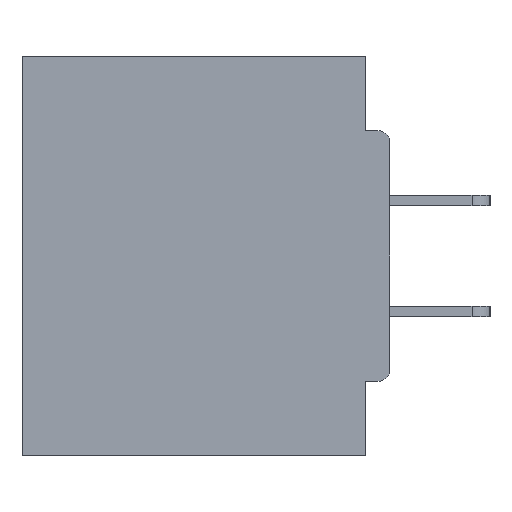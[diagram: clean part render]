
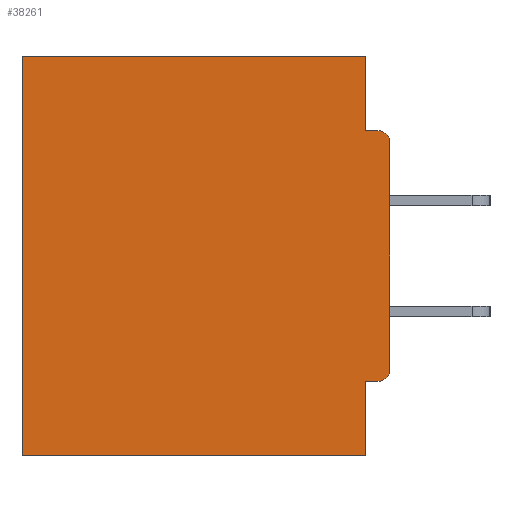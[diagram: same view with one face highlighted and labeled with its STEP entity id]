
A CAD part, left-side view. The second image highlights one B-rep face of the part: STEP entity #38261.
In plain terms, the highlighted planar face has unit normal (-1, 0, 0).
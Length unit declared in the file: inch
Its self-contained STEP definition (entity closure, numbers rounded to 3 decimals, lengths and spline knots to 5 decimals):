
#1 = CARTESIAN_POINT ( 'NONE',  ( 0.298, 0., 0. ) ) ;
#10 = ORIENTED_EDGE ( 'NONE', *, *, #27527, .F. ) ;
#19 = AXIS2_PLACEMENT_3D ( 'NONE', #25079, #4107, #12737 ) ;
#403 = VERTEX_POINT ( 'NONE', #8945 ) ;
#1099 = EDGE_CURVE ( 'NONE', #12573, #403, #3308, .T. ) ;
#2361 = CIRCLE ( 'NONE', #19, 0.015 ) ;
#2599 = VECTOR ( 'NONE', #16436, 39.37008 ) ;
#3308 = LINE ( 'NONE', #29332, #23283 ) ;
#3313 = DIRECTION ( 'NONE',  ( 1., 0., 0. ) ) ;
#4107 = DIRECTION ( 'NONE',  ( -1., 0., 0. ) ) ;
#4191 = LINE ( 'NONE', #11515, #24148 ) ;
#4206 = CARTESIAN_POINT ( 'NONE',  ( 0.298, 0.031, -0.4065 ) ) ;
#4776 = DIRECTION ( 'NONE',  ( 0., 0., -1. ) ) ;
#4802 = DIRECTION ( 'NONE',  ( -1., 0., 0. ) ) ;
#5469 = ORIENTED_EDGE ( 'NONE', *, *, #5647, .T. ) ;
#5568 = LINE ( 'NONE', #31179, #26936 ) ;
#5587 = VERTEX_POINT ( 'NONE', #21786 ) ;
#5647 = EDGE_CURVE ( 'NONE', #19175, #5587, #13406, .T. ) ;
#5949 = LINE ( 'NONE', #16168, #2599 ) ;
#6854 = ORIENTED_EDGE ( 'NONE', *, *, #15138, .T. ) ;
#6889 = DIRECTION ( 'NONE',  ( 0., 1., 0. ) ) ;
#8459 = DIRECTION ( 'NONE',  ( 0., 1., 0. ) ) ;
#8945 = CARTESIAN_POINT ( 'NONE',  ( 0.298, 0.031, -0.5 ) ) ;
#9092 = EDGE_CURVE ( 'NONE', #21730, #30964, #26271, .T. ) ;
#9103 = LINE ( 'NONE', #19027, #26215 ) ;
#9618 = CARTESIAN_POINT ( 'NONE',  ( 0.298, 0., 0. ) ) ;
#9807 = CARTESIAN_POINT ( 'NONE',  ( 0.298, 0.46, -0.5 ) ) ;
#10037 = CARTESIAN_POINT ( 'NONE',  ( 0.298, 0., -0.3915 ) ) ;
#10642 = VECTOR ( 'NONE', #24875, 39.37008 ) ;
#11515 = CARTESIAN_POINT ( 'NONE',  ( 0.298, 0., -0.5 ) ) ;
#11599 = EDGE_CURVE ( 'NONE', #403, #28120, #4191, .T. ) ;
#12137 = CARTESIAN_POINT ( 'NONE',  ( 0.298, 0.015, -0.0935 ) ) ;
#12368 = CARTESIAN_POINT ( 'NONE',  ( 0.298, 0.031, -0.0935 ) ) ;
#12519 = CARTESIAN_POINT ( 'NONE',  ( 0.298, 0.031, -0.5 ) ) ;
#12573 = VERTEX_POINT ( 'NONE', #4206 ) ;
#12737 = DIRECTION ( 'NONE',  ( 0., 0., -1. ) ) ;
#13051 = CARTESIAN_POINT ( 'NONE',  ( 0.298, 0.015, -0.4065 ) ) ;
#13172 = EDGE_CURVE ( 'NONE', #37526, #30964, #5568, .T. ) ;
#13406 = LINE ( 'NONE', #15814, #27646 ) ;
#13421 = ORIENTED_EDGE ( 'NONE', *, *, #32787, .F. ) ;
#14920 = LINE ( 'NONE', #12519, #10642 ) ;
#15113 = DIRECTION ( 'NONE',  ( 0., 0., -1. ) ) ;
#15138 = EDGE_CURVE ( 'NONE', #5587, #28120, #5949, .T. ) ;
#15471 = ORIENTED_EDGE ( 'NONE', *, *, #11599, .F. ) ;
#15814 = CARTESIAN_POINT ( 'NONE',  ( 0.298, 0., 0. ) ) ;
#16168 = CARTESIAN_POINT ( 'NONE',  ( 0.298, 0.46, 0. ) ) ;
#16307 = DIRECTION ( 'NONE',  ( 0., -1., 0. ) ) ;
#16319 = ORIENTED_EDGE ( 'NONE', *, *, #1099, .F. ) ;
#16436 = DIRECTION ( 'NONE',  ( 0., 0., -1. ) ) ;
#18049 = PLANE ( 'NONE',  #19138 ) ;
#18093 = ORIENTED_EDGE ( 'NONE', *, *, #9092, .T. ) ;
#18647 = FACE_OUTER_BOUND ( 'NONE', #21057, .T. ) ;
#19027 = CARTESIAN_POINT ( 'NONE',  ( 0.298, 0., -0.4065 ) ) ;
#19138 = AXIS2_PLACEMENT_3D ( 'NONE', #1, #3313, #15113 ) ;
#19175 = VERTEX_POINT ( 'NONE', #28108 ) ;
#19326 = VECTOR ( 'NONE', #24627, 39.37008 ) ;
#21057 = EDGE_LOOP ( 'NONE', ( #18093, #24665, #13421, #5469, #6854, #15471, #16319, #10, #34621, #32211 ) ) ;
#21522 = VERTEX_POINT ( 'NONE', #10037 ) ;
#21730 = VERTEX_POINT ( 'NONE', #32889 ) ;
#21786 = CARTESIAN_POINT ( 'NONE',  ( 0.298, 0.46, 0. ) ) ;
#23283 = VECTOR ( 'NONE', #4776, 39.37008 ) ;
#24148 = VECTOR ( 'NONE', #8459, 39.37008 ) ;
#24627 = DIRECTION ( 'NONE',  ( 0., 0., -1. ) ) ;
#24665 = ORIENTED_EDGE ( 'NONE', *, *, #13172, .F. ) ;
#24875 = DIRECTION ( 'NONE',  ( 0., 0., -1. ) ) ;
#25079 = CARTESIAN_POINT ( 'NONE',  ( 0.298, 0.015, -0.3915 ) ) ;
#26007 = LINE ( 'NONE', #9618, #19326 ) ;
#26215 = VECTOR ( 'NONE', #36690, 39.37008 ) ;
#26271 = CIRCLE ( 'NONE', #37431, 0.015 ) ;
#26512 = EDGE_CURVE ( 'NONE', #27689, #21522, #2361, .T. ) ;
#26936 = VECTOR ( 'NONE', #16307, 39.37008 ) ;
#27527 = EDGE_CURVE ( 'NONE', #27689, #12573, #9103, .T. ) ;
#27646 = VECTOR ( 'NONE', #6889, 39.37008 ) ;
#27689 = VERTEX_POINT ( 'NONE', #13051 ) ;
#28108 = CARTESIAN_POINT ( 'NONE',  ( 0.298, 0.031, 0. ) ) ;
#28120 = VERTEX_POINT ( 'NONE', #9807 ) ;
#29332 = CARTESIAN_POINT ( 'NONE',  ( 0.298, 0.031, -0.5 ) ) ;
#30964 = VERTEX_POINT ( 'NONE', #12137 ) ;
#31084 = EDGE_CURVE ( 'NONE', #21730, #21522, #26007, .T. ) ;
#31179 = CARTESIAN_POINT ( 'NONE',  ( 0.298, 0., -0.0935 ) ) ;
#32211 = ORIENTED_EDGE ( 'NONE', *, *, #31084, .F. ) ;
#32787 = EDGE_CURVE ( 'NONE', #19175, #37526, #14920, .T. ) ;
#32889 = CARTESIAN_POINT ( 'NONE',  ( 0.298, 0., -0.1085 ) ) ;
#34621 = ORIENTED_EDGE ( 'NONE', *, *, #26512, .T. ) ;
#35203 = DIRECTION ( 'NONE',  ( 0., 0., -1. ) ) ;
#36690 = DIRECTION ( 'NONE',  ( 0., 1., 0. ) ) ;
#37431 = AXIS2_PLACEMENT_3D ( 'NONE', #38095, #4802, #35203 ) ;
#37526 = VERTEX_POINT ( 'NONE', #12368 ) ;
#38095 = CARTESIAN_POINT ( 'NONE',  ( 0.298, 0.015, -0.1085 ) ) ;
#38261 = ADVANCED_FACE ( 'NONE', ( #18647 ), #18049, .F. ) ;
